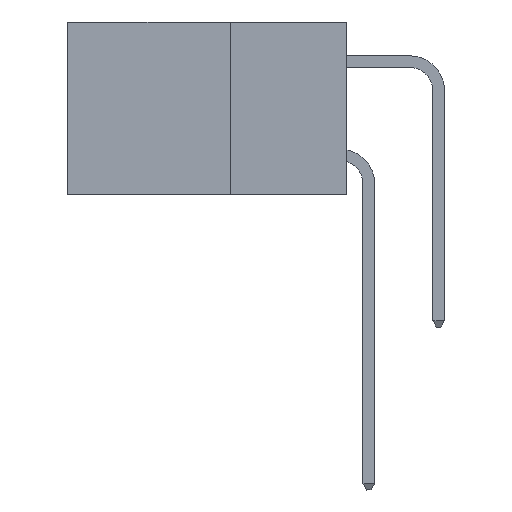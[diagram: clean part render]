
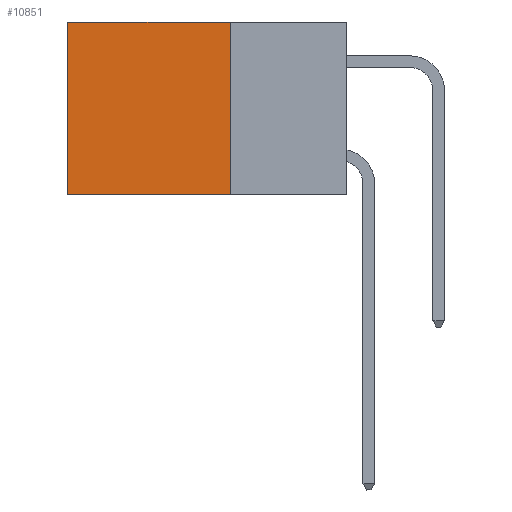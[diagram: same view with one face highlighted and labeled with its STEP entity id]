
A CAD part, left-side view. The second image highlights one B-rep face of the part: STEP entity #10851.
In plain terms, the highlighted planar face has unit normal (-1, 0, 0).
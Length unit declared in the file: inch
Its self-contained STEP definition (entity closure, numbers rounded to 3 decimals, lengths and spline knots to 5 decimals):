
#1260 = CARTESIAN_POINT ( 'NONE',  ( 0.2875, 0.25, 0. ) ) ;
#1326 = DIRECTION ( 'NONE',  ( 0., 0., -1. ) ) ;
#1868 = DIRECTION ( 'NONE',  ( 0., 0., -1. ) ) ;
#3428 = DIRECTION ( 'NONE',  ( 0., 1., 0. ) ) ;
#3523 = ORIENTED_EDGE ( 'NONE', *, *, #7507, .T. ) ;
#3803 = DIRECTION ( 'NONE',  ( 1., 0., 0. ) ) ;
#3918 = VECTOR ( 'NONE', #13611, 39.37008 ) ;
#4258 = VERTEX_POINT ( 'NONE', #4383 ) ;
#4274 = CARTESIAN_POINT ( 'NONE',  ( 0.2875, 0.25, -0.37 ) ) ;
#4383 = CARTESIAN_POINT ( 'NONE',  ( 0.2875, 0.25, -0.37 ) ) ;
#4413 = ORIENTED_EDGE ( 'NONE', *, *, #6004, .F. ) ;
#4483 = CARTESIAN_POINT ( 'NONE',  ( 0.2875, 0.6, 0. ) ) ;
#4742 = CARTESIAN_POINT ( 'NONE',  ( 0.2875, 0.25, 0. ) ) ;
#4751 = EDGE_CURVE ( 'NONE', #10145, #6105, #5221, .T. ) ;
#4903 = PLANE ( 'NONE',  #12101 ) ;
#5221 = LINE ( 'NONE', #4483, #12574 ) ;
#6004 = EDGE_CURVE ( 'NONE', #4258, #6105, #6585, .T. ) ;
#6105 = VERTEX_POINT ( 'NONE', #7054 ) ;
#6585 = LINE ( 'NONE', #4274, #9582 ) ;
#7054 = CARTESIAN_POINT ( 'NONE',  ( 0.2875, 0.6, -0.37 ) ) ;
#7507 = EDGE_CURVE ( 'NONE', #12219, #10145, #16227, .T. ) ;
#8888 = DIRECTION ( 'NONE',  ( 0., 0., -1. ) ) ;
#9169 = VECTOR ( 'NONE', #8888, 39.37008 ) ;
#9582 = VECTOR ( 'NONE', #3428, 39.37008 ) ;
#10145 = VERTEX_POINT ( 'NONE', #13408 ) ;
#10371 = CARTESIAN_POINT ( 'NONE',  ( 0.2875, 0.25, 0. ) ) ;
#10851 = ADVANCED_FACE ( 'NONE', ( #15847 ), #4903, .F. ) ;
#10950 = LINE ( 'NONE', #15044, #9169 ) ;
#11040 = ORIENTED_EDGE ( 'NONE', *, *, #4751, .T. ) ;
#12101 = AXIS2_PLACEMENT_3D ( 'NONE', #1260, #3803, #1326 ) ;
#12219 = VERTEX_POINT ( 'NONE', #10371 ) ;
#12416 = ORIENTED_EDGE ( 'NONE', *, *, #15912, .F. ) ;
#12574 = VECTOR ( 'NONE', #1868, 39.37008 ) ;
#13408 = CARTESIAN_POINT ( 'NONE',  ( 0.2875, 0.6, 0. ) ) ;
#13611 = DIRECTION ( 'NONE',  ( 0., 1., 0. ) ) ;
#14518 = EDGE_LOOP ( 'NONE', ( #11040, #4413, #12416, #3523 ) ) ;
#15044 = CARTESIAN_POINT ( 'NONE',  ( 0.2875, 0.25, 0. ) ) ;
#15847 = FACE_OUTER_BOUND ( 'NONE', #14518, .T. ) ;
#15912 = EDGE_CURVE ( 'NONE', #12219, #4258, #10950, .T. ) ;
#16227 = LINE ( 'NONE', #4742, #3918 ) ;
